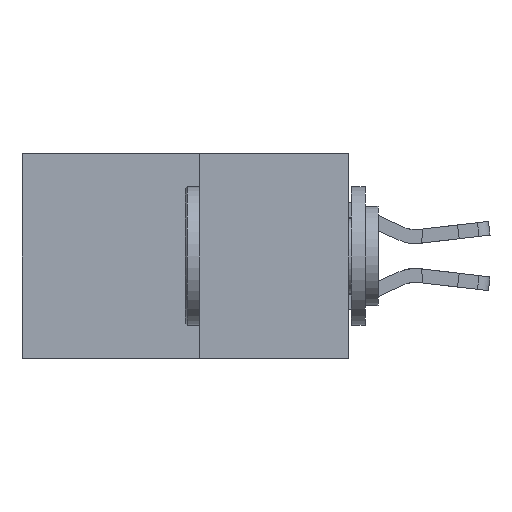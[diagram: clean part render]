
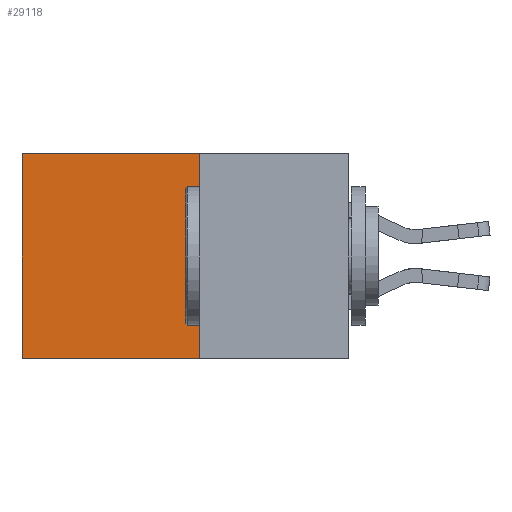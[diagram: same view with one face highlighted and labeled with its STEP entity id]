
A CAD part, left-side view. The second image highlights one B-rep face of the part: STEP entity #29118.
In plain terms, the highlighted planar face has unit normal (-1, 0, 0).
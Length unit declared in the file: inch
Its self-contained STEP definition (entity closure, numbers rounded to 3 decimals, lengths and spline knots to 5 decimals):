
#982 = LINE ( 'NONE', #29516, #12023 ) ;
#2842 = VERTEX_POINT ( 'NONE', #19021 ) ;
#3591 = VECTOR ( 'NONE', #23114, 39.37008 ) ;
#4084 = EDGE_CURVE ( 'NONE', #4714, #2842, #21162, .T. ) ;
#4225 = DIRECTION ( 'NONE',  ( 0., 0., -1. ) ) ;
#4534 = CARTESIAN_POINT ( 'NONE',  ( 0.277, 0.27, -0.37 ) ) ;
#4714 = VERTEX_POINT ( 'NONE', #28070 ) ;
#4741 = DIRECTION ( 'NONE',  ( 0., 0., -1. ) ) ;
#5146 = EDGE_LOOP ( 'NONE', ( #14232, #15812, #17875, #29116 ) ) ;
#5707 = VECTOR ( 'NONE', #26400, 39.37008 ) ;
#5956 = CARTESIAN_POINT ( 'NONE',  ( 0.277, 0.27, -0.37 ) ) ;
#6314 = AXIS2_PLACEMENT_3D ( 'NONE', #16416, #18716, #4741 ) ;
#8762 = VECTOR ( 'NONE', #10034, 39.37008 ) ;
#9469 = FACE_OUTER_BOUND ( 'NONE', #5146, .T. ) ;
#9808 = LINE ( 'NONE', #4534, #3591 ) ;
#10034 = DIRECTION ( 'NONE',  ( 0., 1., 0. ) ) ;
#10179 = CARTESIAN_POINT ( 'NONE',  ( 0.277, 0.27, 0. ) ) ;
#12023 = VECTOR ( 'NONE', #4225, 39.37008 ) ;
#14232 = ORIENTED_EDGE ( 'NONE', *, *, #22568, .T. ) ;
#15812 = ORIENTED_EDGE ( 'NONE', *, *, #16846, .F. ) ;
#16416 = CARTESIAN_POINT ( 'NONE',  ( 0.277, 0.27, -0.37 ) ) ;
#16526 = PLANE ( 'NONE',  #6314 ) ;
#16764 = EDGE_CURVE ( 'NONE', #4714, #20662, #982, .T. ) ;
#16846 = EDGE_CURVE ( 'NONE', #20662, #21889, #9808, .T. ) ;
#17175 = CARTESIAN_POINT ( 'NONE',  ( 0.277, 0.59, -0.37 ) ) ;
#17875 = ORIENTED_EDGE ( 'NONE', *, *, #16764, .F. ) ;
#18716 = DIRECTION ( 'NONE',  ( 1., 0., 0. ) ) ;
#19021 = CARTESIAN_POINT ( 'NONE',  ( 0.277, 0.59, 0. ) ) ;
#20662 = VERTEX_POINT ( 'NONE', #5956 ) ;
#21162 = LINE ( 'NONE', #10179, #8762 ) ;
#21889 = VERTEX_POINT ( 'NONE', #17175 ) ;
#22568 = EDGE_CURVE ( 'NONE', #2842, #21889, #24212, .T. ) ;
#23114 = DIRECTION ( 'NONE',  ( 0., 1., 0. ) ) ;
#24149 = CARTESIAN_POINT ( 'NONE',  ( 0.277, 0.59, -0.37 ) ) ;
#24212 = LINE ( 'NONE', #24149, #5707 ) ;
#26400 = DIRECTION ( 'NONE',  ( 0., 0., -1. ) ) ;
#28070 = CARTESIAN_POINT ( 'NONE',  ( 0.277, 0.27, 0. ) ) ;
#29116 = ORIENTED_EDGE ( 'NONE', *, *, #4084, .T. ) ;
#29118 = ADVANCED_FACE ( 'NONE', ( #9469 ), #16526, .F. ) ;
#29516 = CARTESIAN_POINT ( 'NONE',  ( 0.277, 0.27, -0.37 ) ) ;
